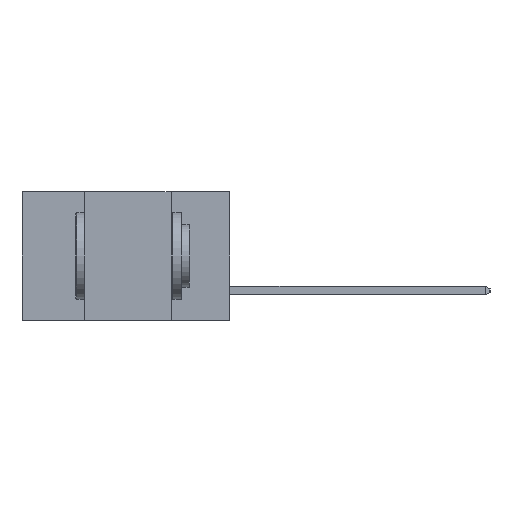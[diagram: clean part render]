
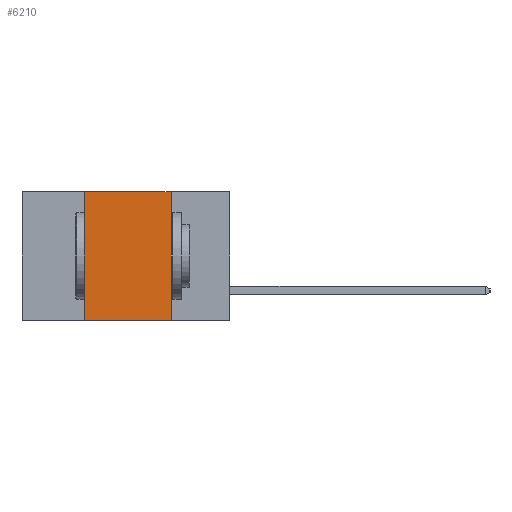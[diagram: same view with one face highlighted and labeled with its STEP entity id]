
A CAD part, left-side view. The second image highlights one B-rep face of the part: STEP entity #6210.
In plain terms, the highlighted planar face has unit normal (-1, 0, 0).
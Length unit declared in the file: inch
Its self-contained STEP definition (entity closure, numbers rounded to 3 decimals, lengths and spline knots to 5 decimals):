
#12 = EDGE_CURVE ( 'NONE', #5299, #11803, #15827, .T. ) ;
#305 = LINE ( 'NONE', #16707, #8282 ) ;
#3149 = CARTESIAN_POINT ( 'NONE',  ( 0., 0.42, 0. ) ) ;
#3176 = CARTESIAN_POINT ( 'NONE',  ( 0., 0.42, 0. ) ) ;
#3582 = EDGE_CURVE ( 'NONE', #16304, #11803, #305, .T. ) ;
#3660 = CARTESIAN_POINT ( 'NONE',  ( 0., 0.17, -0.37 ) ) ;
#4818 = DIRECTION ( 'NONE',  ( 0., 0., 1. ) ) ;
#5084 = ORIENTED_EDGE ( 'NONE', *, *, #12, .T. ) ;
#5299 = VERTEX_POINT ( 'NONE', #11958 ) ;
#5952 = DIRECTION ( 'NONE',  ( 0., -1., 0. ) ) ;
#6210 = ADVANCED_FACE ( 'NONE', ( #14202 ), #11536, .F. ) ;
#6771 = LINE ( 'NONE', #16803, #10418 ) ;
#7776 = ORIENTED_EDGE ( 'NONE', *, *, #3582, .F. ) ;
#7895 = CARTESIAN_POINT ( 'NONE',  ( 0., 0.17, 0. ) ) ;
#8282 = VECTOR ( 'NONE', #11290, 39.37008 ) ;
#10418 = VECTOR ( 'NONE', #5952, 39.37008 ) ;
#11290 = DIRECTION ( 'NONE',  ( 0., 0., -1. ) ) ;
#11536 = PLANE ( 'NONE',  #14525 ) ;
#11539 = EDGE_LOOP ( 'NONE', ( #7776, #16002, #12345, #5084 ) ) ;
#11698 = VECTOR ( 'NONE', #12563, 39.37008 ) ;
#11710 = CARTESIAN_POINT ( 'NONE',  ( 0., 0.6, 0. ) ) ;
#11803 = VERTEX_POINT ( 'NONE', #3660 ) ;
#11958 = CARTESIAN_POINT ( 'NONE',  ( 0., 0.42, -0.37 ) ) ;
#12345 = ORIENTED_EDGE ( 'NONE', *, *, #14352, .F. ) ;
#12563 = DIRECTION ( 'NONE',  ( 0., -1., 0. ) ) ;
#13847 = CARTESIAN_POINT ( 'NONE',  ( 0., 0.6, -0.37 ) ) ;
#14202 = FACE_OUTER_BOUND ( 'NONE', #11539, .T. ) ;
#14352 = EDGE_CURVE ( 'NONE', #5299, #15041, #19848, .T. ) ;
#14525 = AXIS2_PLACEMENT_3D ( 'NONE', #11710, #15602, #15351 ) ;
#15041 = VERTEX_POINT ( 'NONE', #3149 ) ;
#15351 = DIRECTION ( 'NONE',  ( 0., 0., -1. ) ) ;
#15602 = DIRECTION ( 'NONE',  ( 1., 0., 0. ) ) ;
#15827 = LINE ( 'NONE', #13847, #11698 ) ;
#15839 = VECTOR ( 'NONE', #4818, 39.37008 ) ;
#16002 = ORIENTED_EDGE ( 'NONE', *, *, #20130, .F. ) ;
#16304 = VERTEX_POINT ( 'NONE', #7895 ) ;
#16707 = CARTESIAN_POINT ( 'NONE',  ( 0., 0.17, 0. ) ) ;
#16803 = CARTESIAN_POINT ( 'NONE',  ( 0., 0.6, 0. ) ) ;
#19848 = LINE ( 'NONE', #3176, #15839 ) ;
#20130 = EDGE_CURVE ( 'NONE', #15041, #16304, #6771, .T. ) ;
